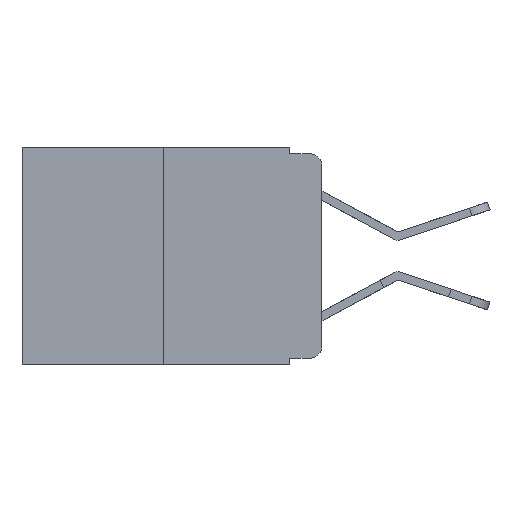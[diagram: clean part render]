
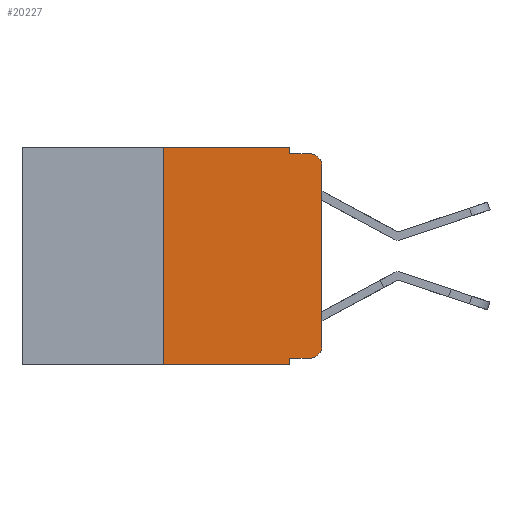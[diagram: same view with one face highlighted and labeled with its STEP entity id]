
A CAD part, left-side view. The second image highlights one B-rep face of the part: STEP entity #20227.
In plain terms, the highlighted planar face has unit normal (-1, 0, 0).
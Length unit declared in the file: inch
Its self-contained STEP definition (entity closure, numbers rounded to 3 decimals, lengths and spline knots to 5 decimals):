
#3 = FACE_OUTER_BOUND ( 'NONE', #12775, .T. ) ;
#599 = EDGE_CURVE ( 'NONE', #24676, #17976, #4808, .T. ) ;
#872 = ORIENTED_EDGE ( 'NONE', *, *, #1446, .F. ) ;
#877 = CARTESIAN_POINT ( 'NONE',  ( 0., 0., -0.313 ) ) ;
#1184 = ORIENTED_EDGE ( 'NONE', *, *, #25422, .T. ) ;
#1228 = EDGE_CURVE ( 'NONE', #4672, #1326, #1894, .T. ) ;
#1326 = VERTEX_POINT ( 'NONE', #14853 ) ;
#1446 = EDGE_CURVE ( 'NONE', #6687, #1326, #4845, .T. ) ;
#1578 = ORIENTED_EDGE ( 'NONE', *, *, #1228, .T. ) ;
#1750 = ORIENTED_EDGE ( 'NONE', *, *, #1880, .T. ) ;
#1880 = EDGE_CURVE ( 'NONE', #5334, #11646, #20343, .T. ) ;
#1894 = LINE ( 'NONE', #12450, #8009 ) ;
#1999 = DIRECTION ( 'NONE',  ( 0., 0., -1. ) ) ;
#2696 = VECTOR ( 'NONE', #12977, 39.37008 ) ;
#3677 = ORIENTED_EDGE ( 'NONE', *, *, #25453, .F. ) ;
#3701 = CARTESIAN_POINT ( 'NONE',  ( 0., 0.051, -0.333 ) ) ;
#4546 = EDGE_CURVE ( 'NONE', #11646, #17055, #25446, .T. ) ;
#4672 = VERTEX_POINT ( 'NONE', #24100 ) ;
#4794 = DIRECTION ( 'NONE',  ( 0., -1., 0. ) ) ;
#4808 = LINE ( 'NONE', #17093, #12194 ) ;
#4845 = LINE ( 'NONE', #19267, #2696 ) ;
#5334 = VERTEX_POINT ( 'NONE', #5451 ) ;
#5344 = AXIS2_PLACEMENT_3D ( 'NONE', #12597, #12735, #23036 ) ;
#5451 = CARTESIAN_POINT ( 'NONE',  ( 0., 0.02, -0.333 ) ) ;
#5699 = LINE ( 'NONE', #22003, #16030 ) ;
#6068 = DIRECTION ( 'NONE',  ( 0., -1., 0. ) ) ;
#6298 = DIRECTION ( 'NONE',  ( 0., -1., 0. ) ) ;
#6300 = EDGE_CURVE ( 'NONE', #17976, #22871, #20825, .T. ) ;
#6543 = CARTESIAN_POINT ( 'NONE',  ( 0., 0.051, 0. ) ) ;
#6687 = VERTEX_POINT ( 'NONE', #3701 ) ;
#7365 = CARTESIAN_POINT ( 'NONE',  ( 0., 0., 0. ) ) ;
#8009 = VECTOR ( 'NONE', #6298, 39.37008 ) ;
#8271 = CARTESIAN_POINT ( 'NONE',  ( 0., 0.473, 0. ) ) ;
#8545 = VECTOR ( 'NONE', #4794, 39.37008 ) ;
#8875 = LINE ( 'NONE', #22928, #21579 ) ;
#9014 = CARTESIAN_POINT ( 'NONE',  ( 0., 0., -0.03 ) ) ;
#9028 = CARTESIAN_POINT ( 'NONE',  ( 0., 0.02, -0.03 ) ) ;
#9550 = DIRECTION ( 'NONE',  ( -1., 0., 0. ) ) ;
#10009 = EDGE_CURVE ( 'NONE', #25628, #24676, #24384, .T. ) ;
#11646 = VERTEX_POINT ( 'NONE', #877 ) ;
#12194 = VECTOR ( 'NONE', #12814, 39.37008 ) ;
#12450 = CARTESIAN_POINT ( 'NONE',  ( 0., 0.473, -0.343 ) ) ;
#12597 = CARTESIAN_POINT ( 'NONE',  ( 0., 0.02, -0.313 ) ) ;
#12735 = DIRECTION ( 'NONE',  ( -1., 0., 0. ) ) ;
#12746 = VECTOR ( 'NONE', #23965, 39.37008 ) ;
#12775 = EDGE_LOOP ( 'NONE', ( #21004, #24598, #17299, #21128, #20658, #3677, #1578, #872, #1184, #1750 ) ) ;
#12814 = DIRECTION ( 'NONE',  ( 0., 0., -1. ) ) ;
#12977 = DIRECTION ( 'NONE',  ( 0., 0., -1. ) ) ;
#14853 = CARTESIAN_POINT ( 'NONE',  ( 0., 0.051, -0.343 ) ) ;
#14891 = AXIS2_PLACEMENT_3D ( 'NONE', #8271, #24591, #1999 ) ;
#15546 = CARTESIAN_POINT ( 'NONE',  ( 0., 0.25, 0. ) ) ;
#16030 = VECTOR ( 'NONE', #16251, 39.37008 ) ;
#16178 = PLANE ( 'NONE',  #14891 ) ;
#16251 = DIRECTION ( 'NONE',  ( 0., -1., 0. ) ) ;
#16686 = CARTESIAN_POINT ( 'NONE',  ( 0., 0.051, -0.01 ) ) ;
#16739 = CARTESIAN_POINT ( 'NONE',  ( 0., 0.02, -0.01 ) ) ;
#17044 = DIRECTION ( 'NONE',  ( 0., 0., 1. ) ) ;
#17055 = VERTEX_POINT ( 'NONE', #9014 ) ;
#17093 = CARTESIAN_POINT ( 'NONE',  ( 0., 0.051, 0. ) ) ;
#17299 = ORIENTED_EDGE ( 'NONE', *, *, #6300, .F. ) ;
#17976 = VERTEX_POINT ( 'NONE', #22751 ) ;
#18366 = CARTESIAN_POINT ( 'NONE',  ( 0., 0.473, 0. ) ) ;
#19267 = CARTESIAN_POINT ( 'NONE',  ( 0., 0.051, 0. ) ) ;
#20227 = ADVANCED_FACE ( 'NONE', ( #3 ), #16178, .F. ) ;
#20343 = CIRCLE ( 'NONE', #5344, 0.02 ) ;
#20658 = ORIENTED_EDGE ( 'NONE', *, *, #10009, .F. ) ;
#20825 = LINE ( 'NONE', #16686, #8545 ) ;
#21004 = ORIENTED_EDGE ( 'NONE', *, *, #4546, .T. ) ;
#21097 = EDGE_CURVE ( 'NONE', #17055, #22871, #23477, .T. ) ;
#21128 = ORIENTED_EDGE ( 'NONE', *, *, #599, .F. ) ;
#21579 = VECTOR ( 'NONE', #17044, 39.37008 ) ;
#22003 = CARTESIAN_POINT ( 'NONE',  ( 0., 0.051, -0.333 ) ) ;
#22751 = CARTESIAN_POINT ( 'NONE',  ( 0., 0.051, -0.01 ) ) ;
#22871 = VERTEX_POINT ( 'NONE', #16739 ) ;
#22928 = CARTESIAN_POINT ( 'NONE',  ( 0., 0.25, 0. ) ) ;
#23036 = DIRECTION ( 'NONE',  ( 0., 0., -1. ) ) ;
#23477 = CIRCLE ( 'NONE', #25192, 0.02 ) ;
#23965 = DIRECTION ( 'NONE',  ( 0., 0., 1. ) ) ;
#24100 = CARTESIAN_POINT ( 'NONE',  ( 0., 0.25, -0.343 ) ) ;
#24315 = VECTOR ( 'NONE', #6068, 39.37008 ) ;
#24384 = LINE ( 'NONE', #18366, #24315 ) ;
#24591 = DIRECTION ( 'NONE',  ( 1., 0., 0. ) ) ;
#24598 = ORIENTED_EDGE ( 'NONE', *, *, #21097, .T. ) ;
#24676 = VERTEX_POINT ( 'NONE', #6543 ) ;
#25192 = AXIS2_PLACEMENT_3D ( 'NONE', #9028, #9550, #25881 ) ;
#25422 = EDGE_CURVE ( 'NONE', #6687, #5334, #5699, .T. ) ;
#25446 = LINE ( 'NONE', #7365, #12746 ) ;
#25453 = EDGE_CURVE ( 'NONE', #4672, #25628, #8875, .T. ) ;
#25628 = VERTEX_POINT ( 'NONE', #15546 ) ;
#25881 = DIRECTION ( 'NONE',  ( 0., 0., -1. ) ) ;
